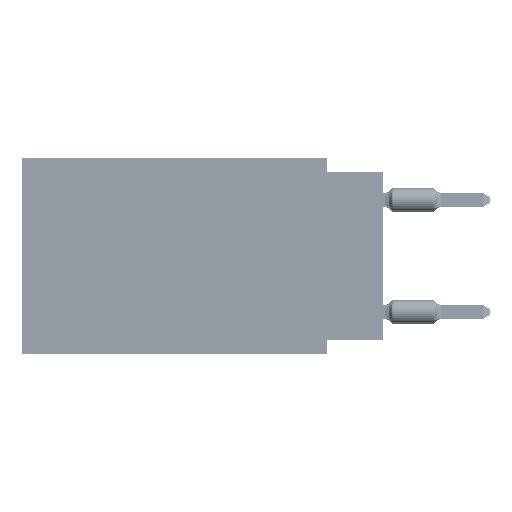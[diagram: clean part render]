
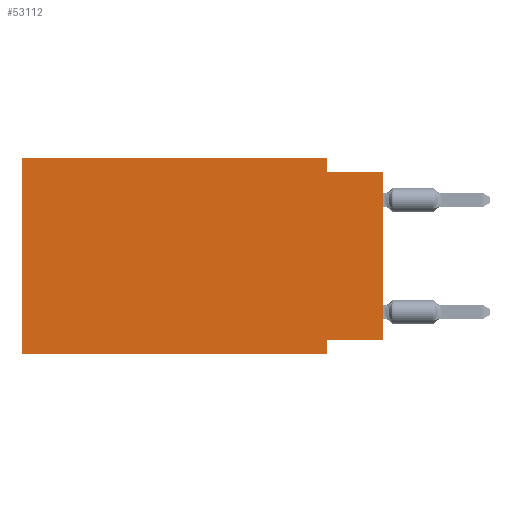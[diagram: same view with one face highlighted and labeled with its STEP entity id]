
A CAD part, left-side view. The second image highlights one B-rep face of the part: STEP entity #53112.
In plain terms, the highlighted planar face has unit normal (-1, 0, 0).
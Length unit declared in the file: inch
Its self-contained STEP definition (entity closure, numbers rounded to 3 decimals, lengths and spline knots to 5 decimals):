
#6 = EDGE_CURVE ( 'NONE', #7144, #12101, #68178, .T. ) ;
#4717 = CARTESIAN_POINT ( 'NONE',  ( 0., 0., -0.325 ) ) ;
#7144 = VERTEX_POINT ( 'NONE', #65362 ) ;
#8734 = DIRECTION ( 'NONE',  ( 0., 0., -1. ) ) ;
#9237 = EDGE_CURVE ( 'NONE', #103066, #100699, #25766, .T. ) ;
#9668 = VECTOR ( 'NONE', #94036, 39.37008 ) ;
#10809 = CARTESIAN_POINT ( 'NONE',  ( 0., 0., -0.325 ) ) ;
#12101 = VERTEX_POINT ( 'NONE', #47809 ) ;
#12705 = LINE ( 'NONE', #4717, #80729 ) ;
#13915 = EDGE_CURVE ( 'NONE', #56505, #18398, #12705, .T. ) ;
#17665 = CARTESIAN_POINT ( 'NONE',  ( 0., 0.1, -0.025 ) ) ;
#18398 = VERTEX_POINT ( 'NONE', #57125 ) ;
#19944 = ORIENTED_EDGE ( 'NONE', *, *, #60908, .T. ) ;
#20038 = CARTESIAN_POINT ( 'NONE',  ( 0., 0., -0.025 ) ) ;
#20617 = CARTESIAN_POINT ( 'NONE',  ( 0., 0.1, -0.35 ) ) ;
#22149 = ORIENTED_EDGE ( 'NONE', *, *, #13915, .F. ) ;
#22865 = CARTESIAN_POINT ( 'NONE',  ( 0., 0.645, -0.35 ) ) ;
#25513 = EDGE_CURVE ( 'NONE', #56505, #100699, #86170, .T. ) ;
#25766 = LINE ( 'NONE', #65119, #36680 ) ;
#27721 = ORIENTED_EDGE ( 'NONE', *, *, #6, .F. ) ;
#33201 = CARTESIAN_POINT ( 'NONE',  ( 0., 0.1, 0. ) ) ;
#34185 = DIRECTION ( 'NONE',  ( 0., 0., 1. ) ) ;
#36680 = VECTOR ( 'NONE', #72035, 39.37008 ) ;
#37171 = DIRECTION ( 'NONE',  ( 0., 1., 0. ) ) ;
#41717 = PLANE ( 'NONE',  #83682 ) ;
#44426 = VECTOR ( 'NONE', #89195, 39.37008 ) ;
#45117 = ORIENTED_EDGE ( 'NONE', *, *, #69631, .F. ) ;
#45692 = CARTESIAN_POINT ( 'NONE',  ( 0., 0.645, 0. ) ) ;
#47809 = CARTESIAN_POINT ( 'NONE',  ( 0., 0.645, 0. ) ) ;
#50052 = VERTEX_POINT ( 'NONE', #20617 ) ;
#50227 = FACE_OUTER_BOUND ( 'NONE', #61688, .T. ) ;
#53112 = ADVANCED_FACE ( 'NONE', ( #50227 ), #41717, .F. ) ;
#53124 = LINE ( 'NONE', #45692, #9668 ) ;
#53752 = CARTESIAN_POINT ( 'NONE',  ( 0., 0., 0. ) ) ;
#55722 = ORIENTED_EDGE ( 'NONE', *, *, #9237, .F. ) ;
#56505 = VERTEX_POINT ( 'NONE', #10809 ) ;
#57125 = CARTESIAN_POINT ( 'NONE',  ( 0., 0.1, -0.325 ) ) ;
#57140 = DIRECTION ( 'NONE',  ( 1., 0., 0. ) ) ;
#60818 = CARTESIAN_POINT ( 'NONE',  ( 0., 0.1, 0. ) ) ;
#60908 = EDGE_CURVE ( 'NONE', #7144, #50052, #95154, .T. ) ;
#61688 = EDGE_LOOP ( 'NONE', ( #74326, #55722, #90556, #70285, #27721, #19944, #45117, #22149 ) ) ;
#65119 = CARTESIAN_POINT ( 'NONE',  ( 0., 0., -0.025 ) ) ;
#65362 = CARTESIAN_POINT ( 'NONE',  ( 0., 0.645, -0.35 ) ) ;
#68178 = LINE ( 'NONE', #83599, #84365 ) ;
#68680 = EDGE_CURVE ( 'NONE', #98141, #103066, #90076, .T. ) ;
#69631 = EDGE_CURVE ( 'NONE', #18398, #50052, #70915, .T. ) ;
#70285 = ORIENTED_EDGE ( 'NONE', *, *, #90702, .F. ) ;
#70915 = LINE ( 'NONE', #103334, #75049 ) ;
#72035 = DIRECTION ( 'NONE',  ( 0., -1., 0. ) ) ;
#74326 = ORIENTED_EDGE ( 'NONE', *, *, #25513, .T. ) ;
#75049 = VECTOR ( 'NONE', #96425, 39.37008 ) ;
#75682 = VECTOR ( 'NONE', #87181, 39.37008 ) ;
#80729 = VECTOR ( 'NONE', #37171, 39.37008 ) ;
#83599 = CARTESIAN_POINT ( 'NONE',  ( 0., 0.645, 0. ) ) ;
#83682 = AXIS2_PLACEMENT_3D ( 'NONE', #89568, #57140, #8734 ) ;
#84365 = VECTOR ( 'NONE', #34185, 39.37008 ) ;
#86170 = LINE ( 'NONE', #53752, #44426 ) ;
#87181 = DIRECTION ( 'NONE',  ( 0., -1., 0. ) ) ;
#89026 = DIRECTION ( 'NONE',  ( 0., 0., -1. ) ) ;
#89195 = DIRECTION ( 'NONE',  ( 0., 0., 1. ) ) ;
#89568 = CARTESIAN_POINT ( 'NONE',  ( 0., 0.645, 0. ) ) ;
#90076 = LINE ( 'NONE', #33201, #103747 ) ;
#90556 = ORIENTED_EDGE ( 'NONE', *, *, #68680, .F. ) ;
#90702 = EDGE_CURVE ( 'NONE', #12101, #98141, #53124, .T. ) ;
#94036 = DIRECTION ( 'NONE',  ( 0., -1., 0. ) ) ;
#95154 = LINE ( 'NONE', #22865, #75682 ) ;
#96425 = DIRECTION ( 'NONE',  ( 0., 0., -1. ) ) ;
#98141 = VERTEX_POINT ( 'NONE', #60818 ) ;
#100699 = VERTEX_POINT ( 'NONE', #20038 ) ;
#103066 = VERTEX_POINT ( 'NONE', #17665 ) ;
#103334 = CARTESIAN_POINT ( 'NONE',  ( 0., 0.1, -0.35 ) ) ;
#103747 = VECTOR ( 'NONE', #89026, 39.37008 ) ;
